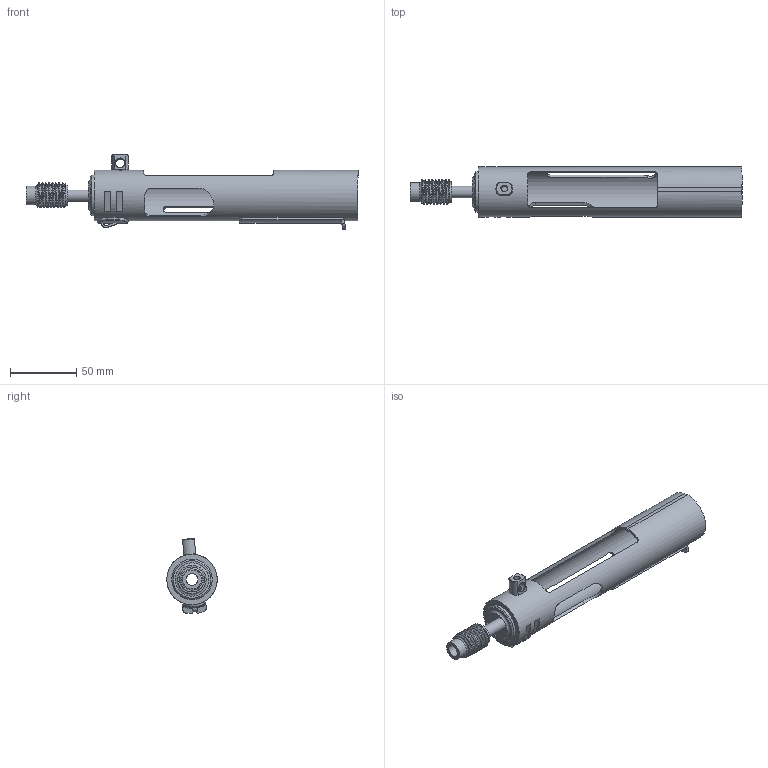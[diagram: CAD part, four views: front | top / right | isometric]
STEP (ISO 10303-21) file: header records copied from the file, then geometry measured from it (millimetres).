
FILE_DESCRIPTION(/* description */ (''),/* implementation_level */ '2;1');
FILE_NAME(/* name */ 'TEC9 Mini Double Stripe (Late Model).step',/* time_stamp */ '2025-06-05T10:03:30-07:00',/* author */ (''),/* organization */ (''),/* preprocessor_version */ 'ST-DEVELOPER v20.1',/* originating_system */ 'Autodesk Translation Framework v14.10.0.0',/* authorisation */ '');
FILE_SCHEMA (('AUTOMOTIVE_DESIGN { 1 0 10303 214 3 1 1 }'));
Length unit declared in the file: millimetre
Products named in the file (1): Mock Up Tec 9
Bounding box: 250.7 x 38.09 x 56.88 mm (x, y, z)
Volume: 53270 mm3; surface area: 50183 mm2
Topology: 6 solids, 6 shells, 140 faces, 384 edges, 261 vertices
Faces by surface type: plane 59, cylinder 57, bspline 14, cone 7, torus 3
Full cylindrical faces by diameter (mm): 5 x2, 7 x1, 8 x1, 9 x2, 14.2 x1, 16.025 x7, 18.885 x8, 30.5 x1, 34.1 x1, 38.1 x1
Entity records: 13730 total; most frequent: CARTESIAN_POINT 10286, ORIENTED_EDGE 768, DIRECTION 605, EDGE_CURVE 384, VERTEX_POINT 261, AXIS2_PLACEMENT_3D 221, EDGE_LOOP 165, LINE 163
